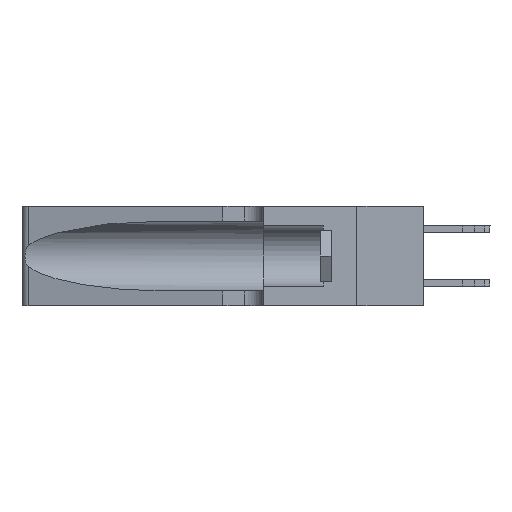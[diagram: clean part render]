
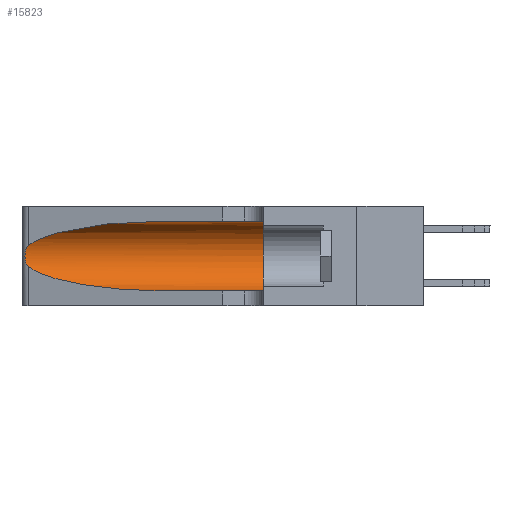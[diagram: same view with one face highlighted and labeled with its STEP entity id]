
A CAD part, left-side view. The second image highlights one B-rep face of the part: STEP entity #15823.
In plain terms, the highlighted cylindrical face has radius 3.308 mm (diameter 6.617 mm), a partial arc.
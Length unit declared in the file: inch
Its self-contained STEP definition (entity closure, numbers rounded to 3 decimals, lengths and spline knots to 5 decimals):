
#288 = DIRECTION ( 'NONE',  ( 0., -1., 0. ) ) ;
#529 = CARTESIAN_POINT ( 'NONE',  ( 0.18966, 0.96281, 0.05475 ) ) ;
#1225 = CARTESIAN_POINT ( 'NONE',  ( 0.25639, 1.23184, 0.21858 ) ) ;
#1592 = CARTESIAN_POINT ( 'NONE',  ( 0.25555, 1.22994, 0.2215 ) ) ;
#2642 =( BOUNDED_CURVE ( )  B_SPLINE_CURVE ( 3, ( #4512, #13160, #19517, #21935 ),
 .UNSPECIFIED., .F., .T. ) 
 B_SPLINE_CURVE_WITH_KNOTS ( ( 4, 4 ),
 ( 1.5708, 2.84003 ),
 .UNSPECIFIED. ) 
 CURVE ( )  GEOMETRIC_REPRESENTATION_ITEM ( )  RATIONAL_B_SPLINE_CURVE ( ( 1., 0.87, 0.87, 1. ) ) 
 REPRESENTATION_ITEM ( '' )  );
#3679 = CIRCLE ( 'NONE', #13891, 0.13025 ) ;
#4366 = CARTESIAN_POINT ( 'NONE',  ( 0.25555, 1.22993, 0.14849 ) ) ;
#4512 = CARTESIAN_POINT ( 'NONE',  ( 0.1305, 0.72297, 0.31525 ) ) ;
#5055 = VECTOR ( 'NONE', #288, 39.37008 ) ;
#5065 = ORIENTED_EDGE ( 'NONE', *, *, #29201, .T. ) ;
#5258 = DIRECTION ( 'NONE',  ( 0., -1., 0. ) ) ;
#5480 = LINE ( 'NONE', #22321, #13456 ) ;
#8272 = VERTEX_POINT ( 'NONE', #9471 ) ;
#8446 = ORIENTED_EDGE ( 'NONE', *, *, #25439, .F. ) ;
#8761 = CARTESIAN_POINT ( 'NONE',  ( 0.2373, 1.15595, 0.08982 ) ) ;
#8890 = CARTESIAN_POINT ( 'NONE',  ( 0.25487, 1.22718, 0.14631 ) ) ;
#9471 = CARTESIAN_POINT ( 'NONE',  ( 0.1305, 0.35, 0.31525 ) ) ;
#9948 = CARTESIAN_POINT ( 'NONE',  ( 0.25856, 1.23593, 0.16098 ) ) ;
#10304 = CARTESIAN_POINT ( 'NONE',  ( 0.25787, 1.23484, 0.2124 ) ) ;
#10878 = ORIENTED_EDGE ( 'NONE', *, *, #32175, .T. ) ;
#13160 = CARTESIAN_POINT ( 'NONE',  ( 0.18966, 0.96281, 0.31525 ) ) ;
#13456 = VECTOR ( 'NONE', #5258, 39.37008 ) ;
#13891 = AXIS2_PLACEMENT_3D ( 'NONE', #21111, #26900, #24142 ) ;
#13925 = CARTESIAN_POINT ( 'NONE',  ( 0.1305, 1.61858, 0.185 ) ) ;
#14379 = CARTESIAN_POINT ( 'NONE',  ( 0.1305, 1.61858, 0.31525 ) ) ;
#15010 = CARTESIAN_POINT ( 'NONE',  ( 0.1305, 0.72297, 0.05475 ) ) ;
#15386 = CARTESIAN_POINT ( 'NONE',  ( 0.1305, 0.72297, 0.31525 ) ) ;
#15524 = CARTESIAN_POINT ( 'NONE',  ( 0.25789, 1.23486, 0.15765 ) ) ;
#15661 = CARTESIAN_POINT ( 'NONE',  ( 0.26018, 1.23835, 0.19895 ) ) ;
#15823 = ADVANCED_FACE ( 'NONE', ( #24604 ), #34465, .F. ) ;
#15906 = CARTESIAN_POINT ( 'NONE',  ( 0.26075, 1.23896, 0.19203 ) ) ;
#16409 = DIRECTION ( 'NONE',  ( 0., 0., -1. ) ) ;
#17701 = ORIENTED_EDGE ( 'NONE', *, *, #25735, .F. ) ;
#18396 = CARTESIAN_POINT ( 'NONE',  ( 0.26075, 1.23896, 0.178 ) ) ;
#19182 = CARTESIAN_POINT ( 'NONE',  ( 0.25487, 1.22718, 0.22369 ) ) ;
#19517 = CARTESIAN_POINT ( 'NONE',  ( 0.2373, 1.15595, 0.28018 ) ) ;
#20241 = EDGE_LOOP ( 'NONE', ( #10878, #5065, #27915, #36346, #17701, #8446 ) ) ;
#20429 = EDGE_CURVE ( 'NONE', #29107, #34667, #5480, .T. ) ;
#21111 = CARTESIAN_POINT ( 'NONE',  ( 0.1305, 0.35, 0.185 ) ) ;
#21549 = CARTESIAN_POINT ( 'NONE',  ( 0.25854, 1.2359, 0.20912 ) ) ;
#21935 = CARTESIAN_POINT ( 'NONE',  ( 0.25487, 1.22718, 0.22369 ) ) ;
#22321 = CARTESIAN_POINT ( 'NONE',  ( 0.1305, 1.61858, 0.05475 ) ) ;
#22521 =( BOUNDED_CURVE ( )  B_SPLINE_CURVE ( 3, ( #8890, #8761, #529, #28765 ),
 .UNSPECIFIED., .F., .F. ) 
 B_SPLINE_CURVE_WITH_KNOTS ( ( 4, 4 ),
 ( 3.44316, 4.71239 ),
 .UNSPECIFIED. ) 
 CURVE ( )  GEOMETRIC_REPRESENTATION_ITEM ( )  RATIONAL_B_SPLINE_CURVE ( ( 1., 0.87, 0.87, 1. ) ) 
 REPRESENTATION_ITEM ( '' )  );
#24048 = CARTESIAN_POINT ( 'NONE',  ( 0.25487, 1.22718, 0.22369 ) ) ;
#24142 = DIRECTION ( 'NONE',  ( 0., 0., 1. ) ) ;
#24402 = CARTESIAN_POINT ( 'NONE',  ( 0.25487, 1.22718, 0.14631 ) ) ;
#24604 = FACE_OUTER_BOUND ( 'NONE', #20241, .T. ) ;
#24758 = VERTEX_POINT ( 'NONE', #15386 ) ;
#25439 = EDGE_CURVE ( 'NONE', #24758, #8272, #36771, .T. ) ;
#25735 = EDGE_CURVE ( 'NONE', #8272, #34667, #3679, .T. ) ;
#26900 = DIRECTION ( 'NONE',  ( 0., 1., 0. ) ) ;
#27316 = CARTESIAN_POINT ( 'NONE',  ( 0.26017, 1.23833, 0.17102 ) ) ;
#27915 = ORIENTED_EDGE ( 'NONE', *, *, #30276, .T. ) ;
#28765 = CARTESIAN_POINT ( 'NONE',  ( 0.1305, 0.72297, 0.05475 ) ) ;
#29107 = VERTEX_POINT ( 'NONE', #15010 ) ;
#29201 = EDGE_CURVE ( 'NONE', #34974, #31566, #33104, .T. ) ;
#29953 = CARTESIAN_POINT ( 'NONE',  ( 0.25639, 1.23186, 0.15144 ) ) ;
#30276 = EDGE_CURVE ( 'NONE', #31566, #29107, #22521, .T. ) ;
#30738 = CARTESIAN_POINT ( 'NONE',  ( 0.25487, 1.22718, 0.14631 ) ) ;
#31566 = VERTEX_POINT ( 'NONE', #30738 ) ;
#32175 = EDGE_CURVE ( 'NONE', #24758, #34974, #2642, .T. ) ;
#32365 = CARTESIAN_POINT ( 'NONE',  ( 0.1305, 0.35, 0.05475 ) ) ;
#33104 = B_SPLINE_CURVE_WITH_KNOTS ( 'NONE', 3,
 ( #24048, #1592, #1225, #10304, #21549, #15661, #15906, #18396, #27316, #9948, #15524, #29953, #4366, #24402 ),
 .UNSPECIFIED., .F., .F.,
 ( 4, 2, 2, 2, 2, 2, 4 ),
 ( 0., 0.00027, 0.00053, 0.00107, 0.0016, 0.00187, 0.00214 ),
 .UNSPECIFIED. ) ;
#33589 = DIRECTION ( 'NONE',  ( 0., -1., 0. ) ) ;
#34465 = CYLINDRICAL_SURFACE ( 'NONE', #35486, 0.13025 ) ;
#34667 = VERTEX_POINT ( 'NONE', #32365 ) ;
#34974 = VERTEX_POINT ( 'NONE', #19182 ) ;
#35486 = AXIS2_PLACEMENT_3D ( 'NONE', #13925, #33589, #16409 ) ;
#36346 = ORIENTED_EDGE ( 'NONE', *, *, #20429, .T. ) ;
#36771 = LINE ( 'NONE', #14379, #5055 ) ;
